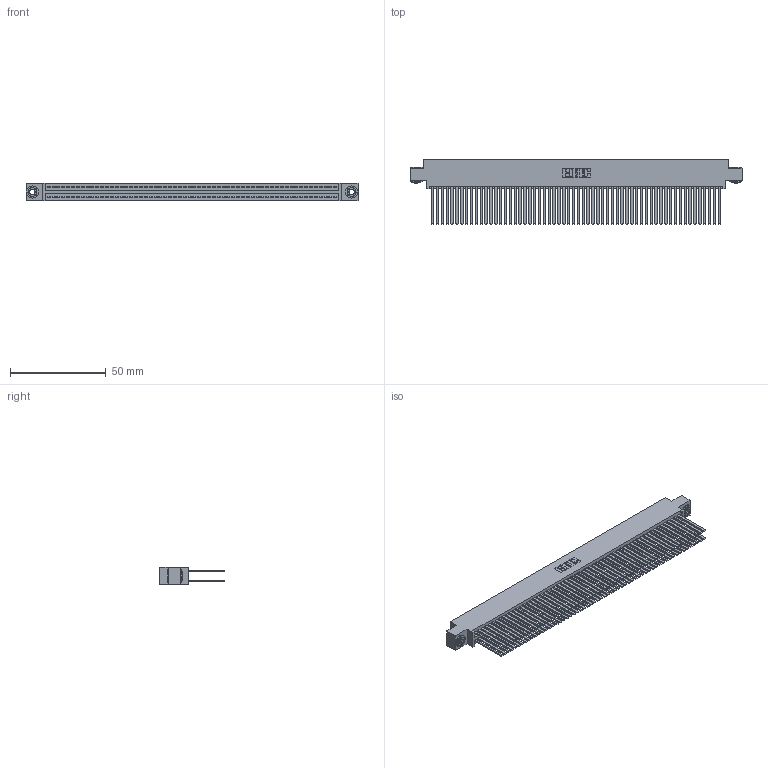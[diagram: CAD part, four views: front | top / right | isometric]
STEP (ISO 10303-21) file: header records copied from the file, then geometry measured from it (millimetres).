
FILE_DESCRIPTION (( 'STEP AP203' ), '1' );
FILE_NAME ('345-120-544-803.STEP', '2019-11-06T02:54:21', ( '' ), ( '' ), 'SwSTEP 2.0', 'SolidWorks 2016', '' );
FILE_SCHEMA (( 'CONFIG_CONTROL_DESIGN' ));
Length unit declared in the file: inch
Products named in the file (4): 345-250-002_345-250-002-102; 345-120-544-803; 345-292-001_345-293-144; 345 Part_0.170 Offset - 0.156 Dia-TH
Assembly tree (123 placements, depth 2):
  345-120-544-803
    345 Part_0.170 Offset - 0.156 Dia-TH
    345-292-001_345-293-144  x120
    345-250-002_345-250-002-102  x2
Bounding box: 173.61 x 33.96 x 9.4 mm (x, y, z)
Volume: 18619.8 mm3; surface area: 33150.5 mm2
Topology: 123 solids, 123 shells, 5448 faces, 16149 edges, 10602 vertices
Faces by surface type: plane 3574, cylinder 1866, cone 8
Entity records: 45252 total; most frequent: CARTESIAN_POINT 7543, ORIENTED_EDGE 7470, DIRECTION 6657, EDGE_CURVE 3735, VECTOR 3343, LINE 3343, VERTEX_POINT 2486, AXIS2_PLACEMENT_3D 1657
